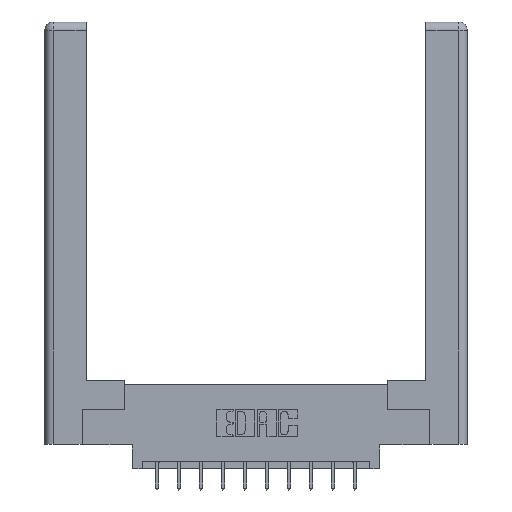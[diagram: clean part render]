
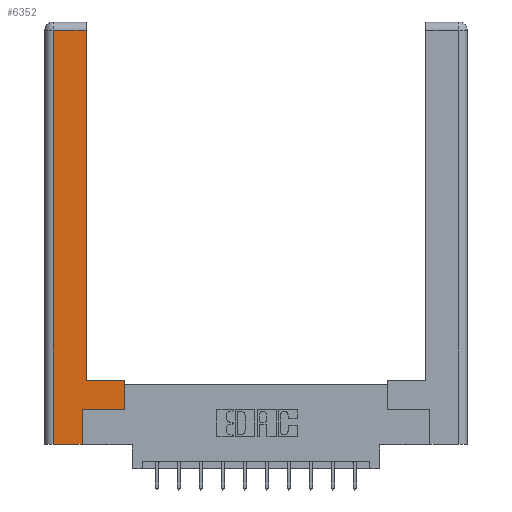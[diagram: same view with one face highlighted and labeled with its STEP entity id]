
A CAD part, top view. The second image highlights one B-rep face of the part: STEP entity #6352.
In plain terms, the highlighted planar face has unit normal (0, 0, 1).
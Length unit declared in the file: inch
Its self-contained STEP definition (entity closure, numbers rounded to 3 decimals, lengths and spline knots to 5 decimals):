
#92 = CARTESIAN_POINT ( 'NONE',  ( 0., 0., 0. ) ) ;
#784 = LINE ( 'NONE', #11218, #9133 ) ;
#964 = VECTOR ( 'NONE', #7901, 39.37008 ) ;
#1147 = ORIENTED_EDGE ( 'NONE', *, *, #6919, .T. ) ;
#1374 = VERTEX_POINT ( 'NONE', #8590 ) ;
#1638 = VERTEX_POINT ( 'NONE', #13771 ) ;
#1838 = FACE_OUTER_BOUND ( 'NONE', #14443, .T. ) ;
#1939 = ORIENTED_EDGE ( 'NONE', *, *, #6971, .T. ) ;
#2109 = CARTESIAN_POINT ( 'NONE',  ( 0.565, 0.45, 0. ) ) ;
#2189 = DIRECTION ( 'NONE',  ( 1., 0., 0. ) ) ;
#2376 = DIRECTION ( 'NONE',  ( -1., 0., 0. ) ) ;
#2514 = AXIS2_PLACEMENT_3D ( 'NONE', #92, #10393, #2376 ) ;
#2934 = ORIENTED_EDGE ( 'NONE', *, *, #10622, .T. ) ;
#3510 = VECTOR ( 'NONE', #10046, 39.37008 ) ;
#3714 = ORIENTED_EDGE ( 'NONE', *, *, #12527, .T. ) ;
#3933 = CARTESIAN_POINT ( 'NONE',  ( 0.565, 0.245, 0. ) ) ;
#3951 = LINE ( 'NONE', #4772, #12312 ) ;
#3966 = VERTEX_POINT ( 'NONE', #14332 ) ;
#4159 = CARTESIAN_POINT ( 'NONE',  ( 0.0615, 2.94, 0. ) ) ;
#4772 = CARTESIAN_POINT ( 'NONE',  ( 0.0615, 0., 0. ) ) ;
#4983 = VECTOR ( 'NONE', #13258, 39.37008 ) ;
#5041 = VERTEX_POINT ( 'NONE', #11778 ) ;
#5495 = CARTESIAN_POINT ( 'NONE',  ( 0.265, 0.245, 0. ) ) ;
#5719 = LINE ( 'NONE', #11109, #4983 ) ;
#5928 = CARTESIAN_POINT ( 'NONE',  ( 0.265, 0.245, 0. ) ) ;
#6062 = ORIENTED_EDGE ( 'NONE', *, *, #11040, .T. ) ;
#6352 = ADVANCED_FACE ( 'NONE', ( #1838 ), #11452, .F. ) ;
#6919 = EDGE_CURVE ( 'NONE', #13618, #14062, #11593, .T. ) ;
#6971 = EDGE_CURVE ( 'NONE', #3966, #1638, #8211, .T. ) ;
#7033 = EDGE_CURVE ( 'NONE', #12330, #1374, #3951, .T. ) ;
#7127 = VECTOR ( 'NONE', #11437, 39.37008 ) ;
#7772 = CARTESIAN_POINT ( 'NONE',  ( 0.295, 3., 0. ) ) ;
#7901 = DIRECTION ( 'NONE',  ( 0., 1., 0. ) ) ;
#8201 = ORIENTED_EDGE ( 'NONE', *, *, #13250, .T. ) ;
#8211 = LINE ( 'NONE', #7772, #11054 ) ;
#8590 = CARTESIAN_POINT ( 'NONE',  ( 0.0615, 0., 0. ) ) ;
#8896 = DIRECTION ( 'NONE',  ( 0., 1., 0. ) ) ;
#9133 = VECTOR ( 'NONE', #2189, 39.37008 ) ;
#9786 = EDGE_CURVE ( 'NONE', #1374, #5041, #12917, .T. ) ;
#10046 = DIRECTION ( 'NONE',  ( 1., 0., 0. ) ) ;
#10278 = CARTESIAN_POINT ( 'NONE',  ( 0.295, 0.45, 0. ) ) ;
#10383 = ORIENTED_EDGE ( 'NONE', *, *, #7033, .T. ) ;
#10393 = DIRECTION ( 'NONE',  ( 0., 0., -1. ) ) ;
#10622 = EDGE_CURVE ( 'NONE', #5041, #11590, #12877, .T. ) ;
#11040 = EDGE_CURVE ( 'NONE', #11590, #13618, #784, .T. ) ;
#11050 = CARTESIAN_POINT ( 'NONE',  ( 0.265, 0., 0. ) ) ;
#11054 = VECTOR ( 'NONE', #11186, 39.37008 ) ;
#11109 = CARTESIAN_POINT ( 'NONE',  ( 0.0615, 2.94, 0. ) ) ;
#11186 = DIRECTION ( 'NONE',  ( 0., 1., 0. ) ) ;
#11218 = CARTESIAN_POINT ( 'NONE',  ( 0.565, 0.245, 0. ) ) ;
#11227 = VECTOR ( 'NONE', #8896, 39.37008 ) ;
#11437 = DIRECTION ( 'NONE',  ( -1., 0., 0. ) ) ;
#11452 = PLANE ( 'NONE',  #2514 ) ;
#11590 = VERTEX_POINT ( 'NONE', #5928 ) ;
#11593 = LINE ( 'NONE', #2109, #11227 ) ;
#11778 = CARTESIAN_POINT ( 'NONE',  ( 0.265, 0., 0. ) ) ;
#11928 = LINE ( 'NONE', #10278, #7127 ) ;
#12312 = VECTOR ( 'NONE', #12908, 39.37008 ) ;
#12330 = VERTEX_POINT ( 'NONE', #4159 ) ;
#12527 = EDGE_CURVE ( 'NONE', #14062, #3966, #11928, .T. ) ;
#12603 = CARTESIAN_POINT ( 'NONE',  ( 0.565, 0.45, 0. ) ) ;
#12694 = ORIENTED_EDGE ( 'NONE', *, *, #9786, .T. ) ;
#12877 = LINE ( 'NONE', #5495, #964 ) ;
#12908 = DIRECTION ( 'NONE',  ( 0., -1., 0. ) ) ;
#12917 = LINE ( 'NONE', #11050, #3510 ) ;
#13250 = EDGE_CURVE ( 'NONE', #1638, #12330, #5719, .T. ) ;
#13258 = DIRECTION ( 'NONE',  ( -1., 0., 0. ) ) ;
#13618 = VERTEX_POINT ( 'NONE', #3933 ) ;
#13771 = CARTESIAN_POINT ( 'NONE',  ( 0.295, 2.94, 0. ) ) ;
#14062 = VERTEX_POINT ( 'NONE', #12603 ) ;
#14332 = CARTESIAN_POINT ( 'NONE',  ( 0.295, 0.45, 0. ) ) ;
#14443 = EDGE_LOOP ( 'NONE', ( #1939, #8201, #10383, #12694, #2934, #6062, #1147, #3714 ) ) ;
